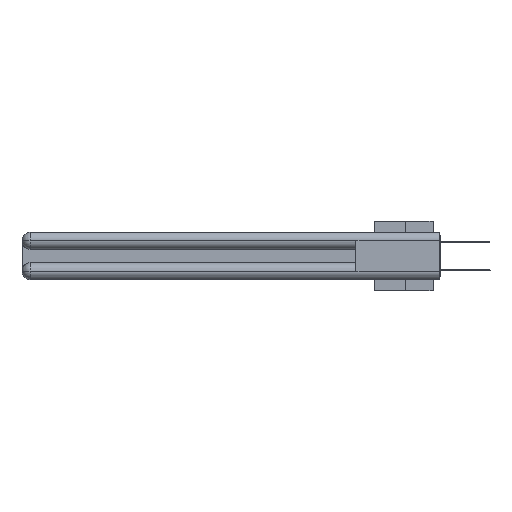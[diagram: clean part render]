
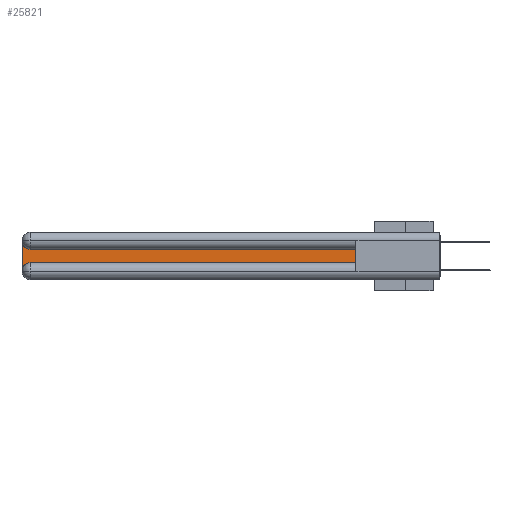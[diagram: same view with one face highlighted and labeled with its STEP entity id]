
A CAD part, left-side view. The second image highlights one B-rep face of the part: STEP entity #25821.
In plain terms, the highlighted planar face has unit normal (-1, 0, 0).
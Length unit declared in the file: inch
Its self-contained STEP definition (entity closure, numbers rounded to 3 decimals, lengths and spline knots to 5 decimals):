
#249 = EDGE_CURVE ( 'NONE', #16101, #15710, #37946, .T. ) ;
#354 = CARTESIAN_POINT ( 'NONE',  ( 0.075, 3., -0.0625 ) ) ;
#642 = CARTESIAN_POINT ( 'NONE',  ( 0.075, 2.94, -0.2775 ) ) ;
#947 = ORIENTED_EDGE ( 'NONE', *, *, #19144, .T. ) ;
#1442 = DIRECTION ( 'NONE',  ( 1., 0., 0. ) ) ;
#2250 = DIRECTION ( 'NONE',  ( 0., 1., 0. ) ) ;
#2784 = EDGE_CURVE ( 'NONE', #15710, #38524, #25357, .T. ) ;
#2801 = CARTESIAN_POINT ( 'NONE',  ( 0.075, 0.6, -0.2175 ) ) ;
#4049 = VECTOR ( 'NONE', #9010, 39.37008 ) ;
#5175 = CARTESIAN_POINT ( 'NONE',  ( 0.075, 2.94, -0.2175 ) ) ;
#6354 = CARTESIAN_POINT ( 'NONE',  ( 0.075, 0.6, -0.2175 ) ) ;
#6576 = EDGE_CURVE ( 'NONE', #38524, #10336, #36438, .T. ) ;
#6724 = DIRECTION ( 'NONE',  ( 1., 0., 0. ) ) ;
#7003 = ORIENTED_EDGE ( 'NONE', *, *, #2784, .T. ) ;
#9010 = DIRECTION ( 'NONE',  ( 0., 0., 1. ) ) ;
#9811 = EDGE_CURVE ( 'NONE', #10336, #22725, #22597, .T. ) ;
#10336 = VERTEX_POINT ( 'NONE', #33342 ) ;
#12555 = VERTEX_POINT ( 'NONE', #20083 ) ;
#14187 = PLANE ( 'NONE',  #25427 ) ;
#14459 = EDGE_CURVE ( 'NONE', #12555, #16101, #19870, .T. ) ;
#15710 = VERTEX_POINT ( 'NONE', #6354 ) ;
#15898 = ORIENTED_EDGE ( 'NONE', *, *, #249, .T. ) ;
#16101 = VERTEX_POINT ( 'NONE', #5175 ) ;
#16537 = CARTESIAN_POINT ( 'NONE',  ( 0.075, 2.94, -0.0625 ) ) ;
#16692 = ORIENTED_EDGE ( 'NONE', *, *, #9811, .T. ) ;
#19144 = EDGE_CURVE ( 'NONE', #22725, #12555, #28762, .T. ) ;
#19425 = CARTESIAN_POINT ( 'NONE',  ( 0.075, 0.6, -0.2175 ) ) ;
#19870 = CIRCLE ( 'NONE', #20006, 0.06 ) ;
#20006 = AXIS2_PLACEMENT_3D ( 'NONE', #642, #6724, #21841 ) ;
#20083 = CARTESIAN_POINT ( 'NONE',  ( 0.075, 3., -0.2775 ) ) ;
#20402 = CARTESIAN_POINT ( 'NONE',  ( 0.075, 0.6, -0.1225 ) ) ;
#21841 = DIRECTION ( 'NONE',  ( 0., 0., -1. ) ) ;
#22597 = CIRCLE ( 'NONE', #39192, 0.06 ) ;
#22660 = DIRECTION ( 'NONE',  ( 0., 0., -1. ) ) ;
#22725 = VERTEX_POINT ( 'NONE', #354 ) ;
#25275 = DIRECTION ( 'NONE',  ( 0., -1., 0. ) ) ;
#25357 = LINE ( 'NONE', #2801, #4049 ) ;
#25427 = AXIS2_PLACEMENT_3D ( 'NONE', #32335, #26289, #29444 ) ;
#25821 = ADVANCED_FACE ( 'NONE', ( #26839 ), #14187, .F. ) ;
#26289 = DIRECTION ( 'NONE',  ( 1., 0., 0. ) ) ;
#26839 = FACE_OUTER_BOUND ( 'NONE', #38495, .T. ) ;
#27187 = CARTESIAN_POINT ( 'NONE',  ( 0.075, 0.6, -0.1225 ) ) ;
#28000 = VECTOR ( 'NONE', #25275, 39.37008 ) ;
#28762 = LINE ( 'NONE', #36386, #36772 ) ;
#29444 = DIRECTION ( 'NONE',  ( 0., 0., -1. ) ) ;
#30061 = DIRECTION ( 'NONE',  ( 0., 0., -1. ) ) ;
#31743 = ORIENTED_EDGE ( 'NONE', *, *, #14459, .T. ) ;
#32335 = CARTESIAN_POINT ( 'NONE',  ( 0.075, 3., -0.1225 ) ) ;
#33342 = CARTESIAN_POINT ( 'NONE',  ( 0.075, 2.94, -0.1225 ) ) ;
#33580 = VECTOR ( 'NONE', #2250, 39.37008 ) ;
#34749 = ORIENTED_EDGE ( 'NONE', *, *, #6576, .T. ) ;
#36386 = CARTESIAN_POINT ( 'NONE',  ( 0.075, 3., -0.2175 ) ) ;
#36438 = LINE ( 'NONE', #20402, #33580 ) ;
#36772 = VECTOR ( 'NONE', #30061, 39.37008 ) ;
#37946 = LINE ( 'NONE', #19425, #28000 ) ;
#38495 = EDGE_LOOP ( 'NONE', ( #34749, #16692, #947, #31743, #15898, #7003 ) ) ;
#38524 = VERTEX_POINT ( 'NONE', #27187 ) ;
#39192 = AXIS2_PLACEMENT_3D ( 'NONE', #16537, #1442, #22660 ) ;
